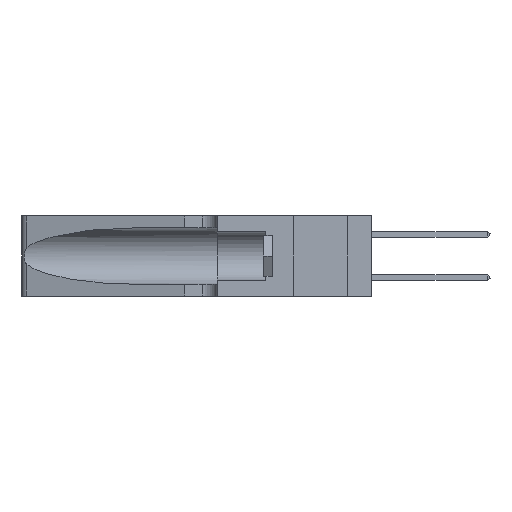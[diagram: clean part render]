
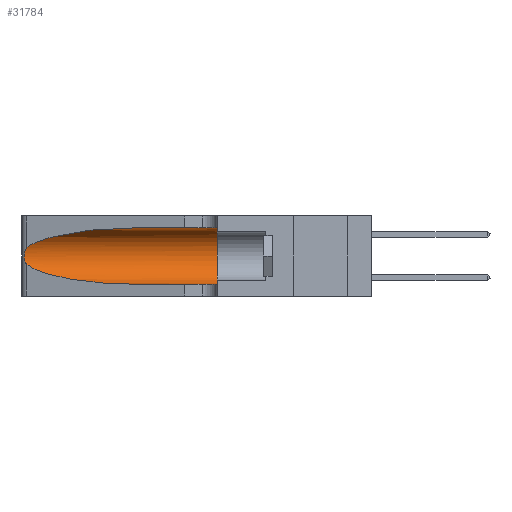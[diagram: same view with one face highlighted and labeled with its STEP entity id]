
A CAD part, left-side view. The second image highlights one B-rep face of the part: STEP entity #31784.
In plain terms, the highlighted cylindrical face has radius 3.308 mm (diameter 6.617 mm), a partial arc.
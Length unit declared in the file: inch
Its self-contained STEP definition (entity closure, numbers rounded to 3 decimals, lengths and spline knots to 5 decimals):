
#733 = CARTESIAN_POINT ( 'NONE',  ( 0.25487, 1.22718, 0.14631 ) ) ;
#1170 = CARTESIAN_POINT ( 'NONE',  ( 0.1305, 1.61858, 0.185 ) ) ;
#1238 =( BOUNDED_CURVE ( )  B_SPLINE_CURVE ( 3, ( #16602, #19530, #1846, #22439 ),
 .UNSPECIFIED., .F., .F. ) 
 B_SPLINE_CURVE_WITH_KNOTS ( ( 4, 4 ),
 ( 1.5708, 2.84003 ),
 .UNSPECIFIED. ) 
 CURVE ( )  GEOMETRIC_REPRESENTATION_ITEM ( )  RATIONAL_B_SPLINE_CURVE ( ( 1., 0.87, 0.87, 1. ) ) 
 REPRESENTATION_ITEM ( '' )  );
#1434 = CARTESIAN_POINT ( 'NONE',  ( 0.1305, 0.35, 0.185 ) ) ;
#1529 = VECTOR ( 'NONE', #5524, 39.37008 ) ;
#1618 = CARTESIAN_POINT ( 'NONE',  ( 0.1305, 0.72297, 0.31525 ) ) ;
#1846 = CARTESIAN_POINT ( 'NONE',  ( 0.2373, 1.15595, 0.28018 ) ) ;
#1943 = EDGE_CURVE ( 'NONE', #13106, #16820, #1238, .T. ) ;
#2031 = EDGE_LOOP ( 'NONE', ( #2709, #34474, #20426, #27244, #10626, #20288 ) ) ;
#2434 = EDGE_CURVE ( 'NONE', #3637, #25012, #30081, .T. ) ;
#2709 = ORIENTED_EDGE ( 'NONE', *, *, #1943, .T. ) ;
#2897 = CARTESIAN_POINT ( 'NONE',  ( 0.1305, 1.61858, 0.05475 ) ) ;
#3550 = VERTEX_POINT ( 'NONE', #733 ) ;
#3637 = VERTEX_POINT ( 'NONE', #30424 ) ;
#4104 = DIRECTION ( 'NONE',  ( 0., -1., 0. ) ) ;
#4324 = AXIS2_PLACEMENT_3D ( 'NONE', #1170, #4104, #33296 ) ;
#4385 = DIRECTION ( 'NONE',  ( 0., 0., 1. ) ) ;
#5205 = CARTESIAN_POINT ( 'NONE',  ( 0.25787, 1.23484, 0.2124 ) ) ;
#5524 = DIRECTION ( 'NONE',  ( 0., -1., 0. ) ) ;
#5712 = CARTESIAN_POINT ( 'NONE',  ( 0.2373, 1.15595, 0.08982 ) ) ;
#8204 = CARTESIAN_POINT ( 'NONE',  ( 0.26018, 1.23835, 0.19895 ) ) ;
#8694 = CARTESIAN_POINT ( 'NONE',  ( 0.25487, 1.22718, 0.14631 ) ) ;
#9805 = VERTEX_POINT ( 'NONE', #20227 ) ;
#10626 = ORIENTED_EDGE ( 'NONE', *, *, #2434, .F. ) ;
#11187 = CARTESIAN_POINT ( 'NONE',  ( 0.26075, 1.23896, 0.178 ) ) ;
#11624 = CARTESIAN_POINT ( 'NONE',  ( 0.1305, 1.61858, 0.31525 ) ) ;
#11672 = CARTESIAN_POINT ( 'NONE',  ( 0.18966, 0.96281, 0.05475 ) ) ;
#11825 = VECTOR ( 'NONE', #26390, 39.37008 ) ;
#13106 = VERTEX_POINT ( 'NONE', #1618 ) ;
#13279 = EDGE_CURVE ( 'NONE', #16820, #3550, #26231, .T. ) ;
#14139 = CARTESIAN_POINT ( 'NONE',  ( 0.25856, 1.23593, 0.16098 ) ) ;
#14620 = AXIS2_PLACEMENT_3D ( 'NONE', #1434, #22037, #4385 ) ;
#16602 = CARTESIAN_POINT ( 'NONE',  ( 0.1305, 0.72297, 0.31525 ) ) ;
#16820 = VERTEX_POINT ( 'NONE', #26980 ) ;
#16973 = CARTESIAN_POINT ( 'NONE',  ( 0.25487, 1.22718, 0.22369 ) ) ;
#17101 = CARTESIAN_POINT ( 'NONE',  ( 0.25639, 1.23186, 0.15144 ) ) ;
#18857 = CYLINDRICAL_SURFACE ( 'NONE', #4324, 0.13025 ) ;
#19530 = CARTESIAN_POINT ( 'NONE',  ( 0.18966, 0.96281, 0.31525 ) ) ;
#19788 = EDGE_CURVE ( 'NONE', #13106, #3637, #32659, .T. ) ;
#20028 = CARTESIAN_POINT ( 'NONE',  ( 0.25487, 1.22718, 0.14631 ) ) ;
#20032 = CARTESIAN_POINT ( 'NONE',  ( 0.1305, 0.35, 0.05475 ) ) ;
#20227 = CARTESIAN_POINT ( 'NONE',  ( 0.1305, 0.72297, 0.05475 ) ) ;
#20288 = ORIENTED_EDGE ( 'NONE', *, *, #19788, .F. ) ;
#20426 = ORIENTED_EDGE ( 'NONE', *, *, #31491, .T. ) ;
#20535 = LINE ( 'NONE', #2897, #11825 ) ;
#22037 = DIRECTION ( 'NONE',  ( 0., 1., 0. ) ) ;
#22439 = CARTESIAN_POINT ( 'NONE',  ( 0.25487, 1.22718, 0.22369 ) ) ;
#22820 = CARTESIAN_POINT ( 'NONE',  ( 0.25639, 1.23184, 0.21858 ) ) ;
#25012 = VERTEX_POINT ( 'NONE', #20032 ) ;
#25730 = CARTESIAN_POINT ( 'NONE',  ( 0.25854, 1.2359, 0.20912 ) ) ;
#26231 = B_SPLINE_CURVE_WITH_KNOTS ( 'NONE', 3,
 ( #16973, #34345, #22820, #5205, #25730, #8204, #28618, #11187, #31544, #14139, #34465, #17101, #37389, #20028 ),
 .UNSPECIFIED., .F., .F.,
 ( 4, 2, 2, 2, 2, 2, 4 ),
 ( 0., 0.00027, 0.00053, 0.00107, 0.0016, 0.00187, 0.00214 ),
 .UNSPECIFIED. ) ;
#26390 = DIRECTION ( 'NONE',  ( 0., -1., 0. ) ) ;
#26819 =( BOUNDED_CURVE ( )  B_SPLINE_CURVE ( 3, ( #8694, #5712, #11672, #32019 ),
 .UNSPECIFIED., .F., .F. ) 
 B_SPLINE_CURVE_WITH_KNOTS ( ( 4, 4 ),
 ( 3.44316, 4.71239 ),
 .UNSPECIFIED. ) 
 CURVE ( )  GEOMETRIC_REPRESENTATION_ITEM ( )  RATIONAL_B_SPLINE_CURVE ( ( 1., 0.87, 0.87, 1. ) ) 
 REPRESENTATION_ITEM ( '' )  );
#26977 = EDGE_CURVE ( 'NONE', #9805, #25012, #20535, .T. ) ;
#26980 = CARTESIAN_POINT ( 'NONE',  ( 0.25487, 1.22718, 0.22369 ) ) ;
#27244 = ORIENTED_EDGE ( 'NONE', *, *, #26977, .T. ) ;
#28618 = CARTESIAN_POINT ( 'NONE',  ( 0.26075, 1.23896, 0.19203 ) ) ;
#30081 = CIRCLE ( 'NONE', #14620, 0.13025 ) ;
#30424 = CARTESIAN_POINT ( 'NONE',  ( 0.1305, 0.35, 0.31525 ) ) ;
#31491 = EDGE_CURVE ( 'NONE', #3550, #9805, #26819, .T. ) ;
#31544 = CARTESIAN_POINT ( 'NONE',  ( 0.26017, 1.23833, 0.17102 ) ) ;
#31784 = ADVANCED_FACE ( 'NONE', ( #34260 ), #18857, .F. ) ;
#32019 = CARTESIAN_POINT ( 'NONE',  ( 0.1305, 0.72297, 0.05475 ) ) ;
#32659 = LINE ( 'NONE', #11624, #1529 ) ;
#33296 = DIRECTION ( 'NONE',  ( 0., 0., -1. ) ) ;
#34260 = FACE_OUTER_BOUND ( 'NONE', #2031, .T. ) ;
#34345 = CARTESIAN_POINT ( 'NONE',  ( 0.25555, 1.22994, 0.2215 ) ) ;
#34465 = CARTESIAN_POINT ( 'NONE',  ( 0.25789, 1.23486, 0.15765 ) ) ;
#34474 = ORIENTED_EDGE ( 'NONE', *, *, #13279, .T. ) ;
#37389 = CARTESIAN_POINT ( 'NONE',  ( 0.25555, 1.22993, 0.14849 ) ) ;
